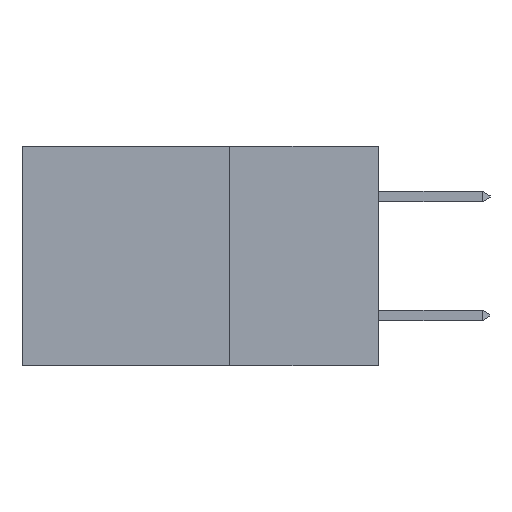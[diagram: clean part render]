
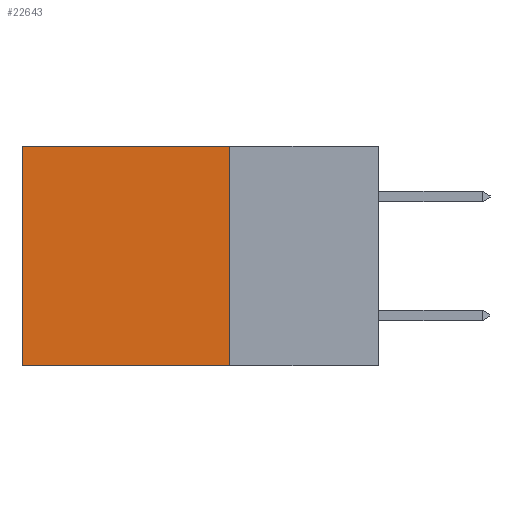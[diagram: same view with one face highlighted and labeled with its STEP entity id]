
A CAD part, left-side view. The second image highlights one B-rep face of the part: STEP entity #22643.
In plain terms, the highlighted planar face has unit normal (-1, 0, 0).
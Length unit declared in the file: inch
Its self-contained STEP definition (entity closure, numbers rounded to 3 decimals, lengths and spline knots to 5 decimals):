
#697 = LINE ( 'NONE', #7516, #6286 ) ;
#1400 = CARTESIAN_POINT ( 'NONE',  ( 0.298, 0.25, 0. ) ) ;
#1674 = VERTEX_POINT ( 'NONE', #1400 ) ;
#1750 = VECTOR ( 'NONE', #22086, 39.37008 ) ;
#1788 = CARTESIAN_POINT ( 'NONE',  ( 0.298, 0.25, 0. ) ) ;
#2042 = CARTESIAN_POINT ( 'NONE',  ( 0.298, 0.6, -0.37 ) ) ;
#4819 = VERTEX_POINT ( 'NONE', #2042 ) ;
#4833 = EDGE_LOOP ( 'NONE', ( #29324, #23780, #26834, #9946 ) ) ;
#5065 = EDGE_CURVE ( 'NONE', #1674, #24700, #697, .T. ) ;
#5498 = CARTESIAN_POINT ( 'NONE',  ( 0.298, 0.25, -0.37 ) ) ;
#5512 = CARTESIAN_POINT ( 'NONE',  ( 0.298, 0.6, 0. ) ) ;
#6015 = CARTESIAN_POINT ( 'NONE',  ( 0.298, 0.25, -0.37 ) ) ;
#6286 = VECTOR ( 'NONE', #19352, 39.37008 ) ;
#6614 = LINE ( 'NONE', #1788, #30261 ) ;
#7081 = VERTEX_POINT ( 'NONE', #6015 ) ;
#7384 = PLANE ( 'NONE',  #10737 ) ;
#7516 = CARTESIAN_POINT ( 'NONE',  ( 0.298, 0.25, 0. ) ) ;
#8090 = DIRECTION ( 'NONE',  ( 0., 0., -1. ) ) ;
#8913 = FACE_OUTER_BOUND ( 'NONE', #4833, .T. ) ;
#9776 = VECTOR ( 'NONE', #8090, 39.37008 ) ;
#9787 = DIRECTION ( 'NONE',  ( 1., 0., 0. ) ) ;
#9946 = ORIENTED_EDGE ( 'NONE', *, *, #5065, .T. ) ;
#10737 = AXIS2_PLACEMENT_3D ( 'NONE', #12084, #9787, #26370 ) ;
#11099 = EDGE_CURVE ( 'NONE', #7081, #4819, #26243, .T. ) ;
#12084 = CARTESIAN_POINT ( 'NONE',  ( 0.298, 0.25, 0. ) ) ;
#13746 = DIRECTION ( 'NONE',  ( 0., 0., -1. ) ) ;
#13956 = EDGE_CURVE ( 'NONE', #24700, #4819, #16090, .T. ) ;
#16090 = LINE ( 'NONE', #19908, #9776 ) ;
#19352 = DIRECTION ( 'NONE',  ( 0., 1., 0. ) ) ;
#19908 = CARTESIAN_POINT ( 'NONE',  ( 0.298, 0.6, 0. ) ) ;
#22086 = DIRECTION ( 'NONE',  ( 0., 1., 0. ) ) ;
#22643 = ADVANCED_FACE ( 'NONE', ( #8913 ), #7384, .F. ) ;
#23780 = ORIENTED_EDGE ( 'NONE', *, *, #11099, .F. ) ;
#24700 = VERTEX_POINT ( 'NONE', #5512 ) ;
#26243 = LINE ( 'NONE', #5498, #1750 ) ;
#26370 = DIRECTION ( 'NONE',  ( 0., 0., -1. ) ) ;
#26834 = ORIENTED_EDGE ( 'NONE', *, *, #28032, .F. ) ;
#28032 = EDGE_CURVE ( 'NONE', #1674, #7081, #6614, .T. ) ;
#29324 = ORIENTED_EDGE ( 'NONE', *, *, #13956, .T. ) ;
#30261 = VECTOR ( 'NONE', #13746, 39.37008 ) ;
